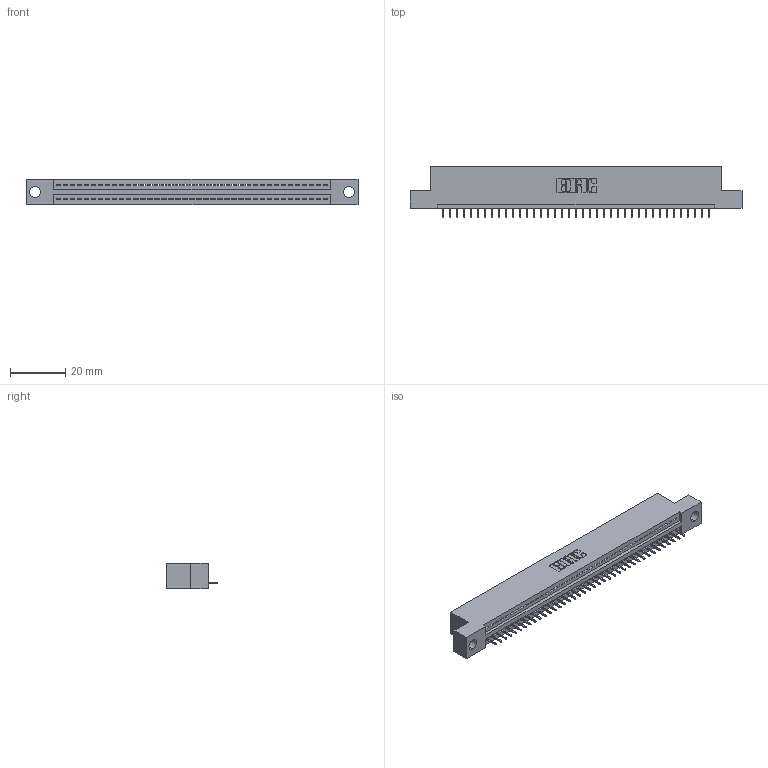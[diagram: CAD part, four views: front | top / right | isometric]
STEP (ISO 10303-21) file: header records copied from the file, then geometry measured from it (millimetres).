
FILE_DESCRIPTION (( 'STEP AP203' ), '1' );
FILE_NAME ('845-039-525-104.STEP', '2020-09-23T04:25:27', ( '' ), ( '' ), 'SwSTEP 2.0', 'SolidWorks 2020', '' );
FILE_SCHEMA (( 'CONFIG_CONTROL_DESIGN' ));
Length unit declared in the file: inch
Products named in the file (3): 845 Part_Flush Mounting Lugs - 0.156 Dia-TH; 345-292-001_345-293-125; 845-039-525-104
Assembly tree (40 placements, depth 2):
  845-039-525-104
    845 Part_Flush Mounting Lugs - 0.156 Dia-TH
    345-292-001_345-293-125  x39
Bounding box: 120.27 x 18.72 x 9.4 mm (x, y, z)
Volume: 11151.6 mm3; surface area: 14056.5 mm2
Topology: 40 solids, 40 shells, 2544 faces, 7361 edges, 4750 vertices
Faces by surface type: plane 1874, cylinder 670
Entity records: 29833 total; most frequent: CARTESIAN_POINT 5173, ORIENTED_EDGE 5146, DIRECTION 4523, EDGE_CURVE 2573, LINE 2289, VECTOR 2289, VERTEX_POINT 1710, AXIS2_PLACEMENT_3D 1117
